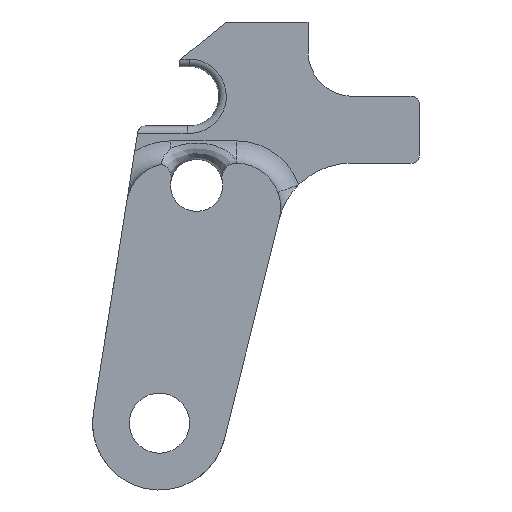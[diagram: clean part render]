
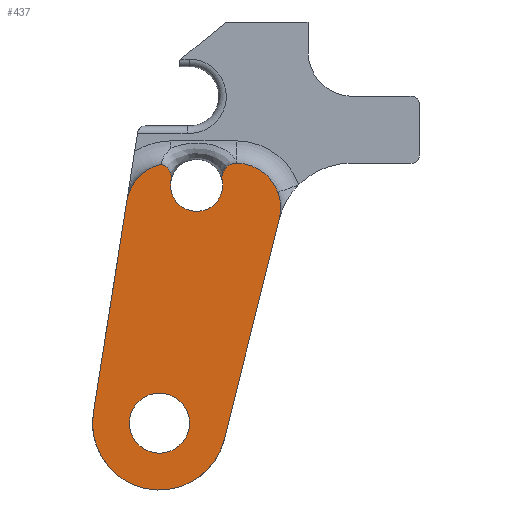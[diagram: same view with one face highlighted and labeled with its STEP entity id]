
A CAD part, left-side view. The second image highlights one B-rep face of the part: STEP entity #437.
In plain terms, the highlighted planar face has unit normal (-1, 0, 0).
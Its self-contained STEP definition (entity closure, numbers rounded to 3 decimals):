
#177=CARTESIAN_POINT('',(-9.0,-10.376,35.));
#178=VERTEX_POINT('',#177);
#244=CARTESIAN_POINT('',(-9.0,-0.302,34.87));
#245=VERTEX_POINT('',#244);
#263=CARTESIAN_POINT('',(-9.0,-1.558,32.636));
#264=VERTEX_POINT('',#263);
#265=CARTESIAN_POINT('',(-9.0,-0.301,34.868));
#266=CARTESIAN_POINT('',(-9.0,-0.543,34.775));
#267=CARTESIAN_POINT('',(-9.0,-0.768,34.637));
#268=CARTESIAN_POINT('',(-9.,-0.957,34.461));
#269=CARTESIAN_POINT('',(-9.,-1.201,34.233));
#270=CARTESIAN_POINT('',(-9.,-1.387,33.942));
#271=CARTESIAN_POINT('',(-9.,-1.491,33.625));
#272=CARTESIAN_POINT('',(-9.,-1.596,33.308));
#273=CARTESIAN_POINT('',(-9.,-1.619,32.965));
#274=CARTESIAN_POINT('',(-9.,-1.558,32.636));
#275=B_SPLINE_CURVE_WITH_KNOTS('',3,(#265,#266,#267,#268,#269,#270,#271,#272,#273,#274),.UNSPECIFIED.,.F.,.U.,(4,3,3,4),(0.073,0.151,0.251,0.352),.UNSPECIFIED.);
#276=EDGE_CURVE('',#245,#264,#275,.T.);
#278=CARTESIAN_POINT('',(-9.,-8.442,32.636));
#279=VERTEX_POINT('',#278);
#301=CARTESIAN_POINT('',(-9.,-8.442,32.636));
#302=CARTESIAN_POINT('',(-9.,-8.381,32.965));
#303=CARTESIAN_POINT('',(-9.,-8.404,33.308));
#304=CARTESIAN_POINT('',(-9.,-8.509,33.625));
#305=CARTESIAN_POINT('',(-9.,-8.613,33.942));
#306=CARTESIAN_POINT('',(-9.,-8.799,34.233));
#307=CARTESIAN_POINT('',(-9.,-9.043,34.461));
#308=CARTESIAN_POINT('',(-9.,-9.401,34.795));
#309=CARTESIAN_POINT('',(-9.,-9.886,34.991));
#310=CARTESIAN_POINT('',(-9.,-10.376,35.));
#311=B_SPLINE_CURVE_WITH_KNOTS('',3,(#301,#302,#303,#304,#305,#306,#307,#308,#309,#310),.UNSPECIFIED.,.F.,.U.,(4,3,3,4),(0.0,0.1,0.201,0.348),.UNSPECIFIED.);
#312=EDGE_CURVE('',#279,#178,#311,.T.);
#323=CARTESIAN_POINT('',(-9.,-15.954,31.066));
#324=VERTEX_POINT('',#323);
#325=CARTESIAN_POINT('',(-9.0,-10.321,29.0));
#326=DIRECTION('',(1.0,0.0,0.0));
#327=DIRECTION('',(0.0,-0.788,0.616));
#328=AXIS2_PLACEMENT_3D('',#325,#326,#327);
#329=CIRCLE('',#328,6.);
#330=EDGE_CURVE('',#178,#324,#329,.T.);
#360=CARTESIAN_POINT('',(-9.0,-5.574,29.918));
#361=DIRECTION('',(1.0,0.0,0.0));
#362=DIRECTION('',(0.0,0.0,-1.0));
#363=AXIS2_PLACEMENT_3D('',#360,#361,#362);
#364=PLANE('',#363);
#365=ORIENTED_EDGE('',*,*,#312,.F.);
#366=CARTESIAN_POINT('',(-9.0,-5.0,32.0));
#367=DIRECTION('',(1.0,0.0,0.0));
#368=DIRECTION('',(0.0,-1.0,0.0));
#369=AXIS2_PLACEMENT_3D('',#366,#367,#368);
#370=CIRCLE('',#369,3.5);
#371=EDGE_CURVE('',#279,#264,#370,.T.);
#372=ORIENTED_EDGE('',*,*,#371,.T.);
#373=ORIENTED_EDGE('',*,*,#276,.F.);
#374=CARTESIAN_POINT('',(-9.0,4.381,29.937));
#375=VERTEX_POINT('',#374);
#376=CARTESIAN_POINT('',(-9.0,-1.546,29.0));
#377=DIRECTION('',(1.0,0.0,0.0));
#378=DIRECTION('',(0.0,0.65,0.76));
#379=AXIS2_PLACEMENT_3D('',#376,#377,#378);
#380=CIRCLE('',#379,6.);
#381=EDGE_CURVE('',#375,#245,#380,.T.);
#382=ORIENTED_EDGE('',*,*,#381,.F.);
#383=CARTESIAN_POINT('',(-9.0,8.89,1.405));
#384=VERTEX_POINT('',#383);
#385=CARTESIAN_POINT('',(-9.0,8.89,1.405));
#386=DIRECTION('',(0.0,-0.156,0.988));
#387=VECTOR('',#386,28.886);
#388=LINE('',#385,#387);
#389=EDGE_CURVE('',#384,#375,#388,.T.);
#390=ORIENTED_EDGE('',*,*,#389,.F.);
#391=CARTESIAN_POINT('',(-9.0,-8.733,-2.177));
#392=VERTEX_POINT('',#391);
#393=CARTESIAN_POINT('',(-9.0,0.0,0.0));
#394=DIRECTION('',(1.0,0.0,0.0));
#395=DIRECTION('',(0.0,1.0,0.0));
#396=AXIS2_PLACEMENT_3D('',#393,#394,#395);
#397=CIRCLE('',#396,9.0);
#398=EDGE_CURVE('',#392,#384,#397,.T.);
#399=ORIENTED_EDGE('',*,*,#398,.F.);
#400=CARTESIAN_POINT('',(-9.,-16.11,27.419));
#401=VERTEX_POINT('',#400);
#402=CARTESIAN_POINT('',(-9.0,-16.11,27.419));
#403=DIRECTION('',(0.0,0.242,-0.97));
#404=VECTOR('',#403,30.501);
#405=LINE('',#402,#404);
#406=EDGE_CURVE('',#401,#392,#405,.T.);
#407=ORIENTED_EDGE('',*,*,#406,.F.);
#408=CARTESIAN_POINT('',(-9.0,-16.143,27.549));
#409=VERTEX_POINT('',#408);
#410=CARTESIAN_POINT('',(-9.0,-16.143,27.549));
#411=DIRECTION('',(0.0,0.242,-0.97));
#412=VECTOR('',#411,0.134);
#413=LINE('',#410,#412);
#414=EDGE_CURVE('',#409,#401,#413,.T.);
#415=ORIENTED_EDGE('',*,*,#414,.F.);
#416=CARTESIAN_POINT('',(-9.0,-10.321,29.0));
#417=DIRECTION('',(1.0,0.0,0.0));
#418=DIRECTION('',(0.0,-0.788,0.616));
#419=AXIS2_PLACEMENT_3D('',#416,#417,#418);
#420=CIRCLE('',#419,6.);
#421=EDGE_CURVE('',#324,#409,#420,.T.);
#422=ORIENTED_EDGE('',*,*,#421,.F.);
#423=ORIENTED_EDGE('',*,*,#330,.F.);
#424=EDGE_LOOP('',(#365,#372,#373,#382,#390,#399,#407,#415,#422,#423));
#425=FACE_OUTER_BOUND('',#424,.T.);
#426=CARTESIAN_POINT('',(-9.0,4.05,0.));
#427=VERTEX_POINT('',#426);
#428=CARTESIAN_POINT('',(-9.0,0.0,0.0));
#429=DIRECTION('',(1.0,0.0,0.0));
#430=DIRECTION('',(0.0,-1.0,0.0));
#431=AXIS2_PLACEMENT_3D('',#428,#429,#430);
#432=CIRCLE('',#431,4.05);
#433=EDGE_CURVE('',#427,#427,#432,.T.);
#434=ORIENTED_EDGE('',*,*,#433,.T.);
#435=EDGE_LOOP('',(#434));
#436=FACE_BOUND('',#435,.T.);
#437=ADVANCED_FACE('',(#425,#436),#364,.F.);
